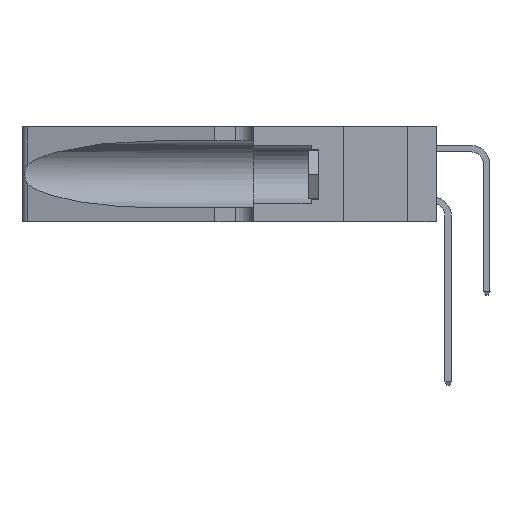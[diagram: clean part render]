
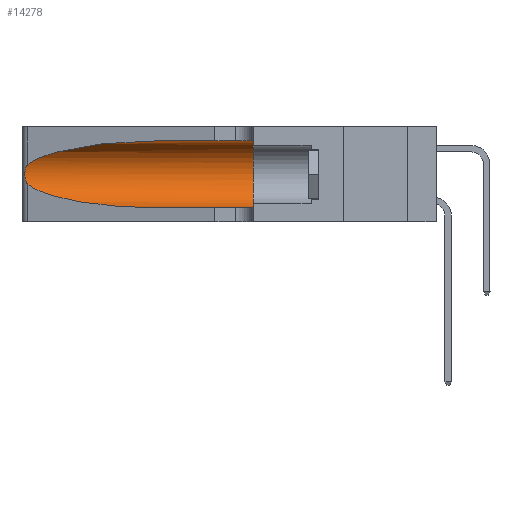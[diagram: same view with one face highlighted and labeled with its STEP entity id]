
A CAD part, left-side view. The second image highlights one B-rep face of the part: STEP entity #14278.
In plain terms, the highlighted cylindrical face has radius 3.308 mm (diameter 6.617 mm), a partial arc.
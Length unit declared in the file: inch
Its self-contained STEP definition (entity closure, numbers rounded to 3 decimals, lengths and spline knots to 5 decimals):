
#244 = CARTESIAN_POINT ( 'NONE',  ( 0.1305, 0.35, 0.31525 ) ) ;
#509 = CARTESIAN_POINT ( 'NONE',  ( 0.1305, 1.61858, 0.31525 ) ) ;
#1307 = CARTESIAN_POINT ( 'NONE',  ( 0.25787, 1.23484, 0.2124 ) ) ;
#2764 = CIRCLE ( 'NONE', #5358, 0.13025 ) ;
#2987 = CARTESIAN_POINT ( 'NONE',  ( 0.25487, 1.22718, 0.22369 ) ) ;
#3011 = DIRECTION ( 'NONE',  ( 0., 0., -1. ) ) ;
#3048 = DIRECTION ( 'NONE',  ( 0., -1., 0. ) ) ;
#3838 = CARTESIAN_POINT ( 'NONE',  ( 0.26018, 1.23835, 0.19895 ) ) ;
#4254 = VECTOR ( 'NONE', #31421, 39.37008 ) ;
#5358 = AXIS2_PLACEMENT_3D ( 'NONE', #22329, #7317, #24875 ) ;
#5828 = CARTESIAN_POINT ( 'NONE',  ( 0.1305, 0.72297, 0.05475 ) ) ;
#6239 = VERTEX_POINT ( 'NONE', #31519 ) ;
#6357 = CARTESIAN_POINT ( 'NONE',  ( 0.26075, 1.23896, 0.178 ) ) ;
#7317 = DIRECTION ( 'NONE',  ( 0., 1., 0. ) ) ;
#7642 = ORIENTED_EDGE ( 'NONE', *, *, #16237, .T. ) ;
#8105 = CARTESIAN_POINT ( 'NONE',  ( 0.25487, 1.22718, 0.14631 ) ) ;
#8329 = VERTEX_POINT ( 'NONE', #24674 ) ;
#8758 = ORIENTED_EDGE ( 'NONE', *, *, #21262, .T. ) ;
#8881 = CARTESIAN_POINT ( 'NONE',  ( 0.25856, 1.23593, 0.16098 ) ) ;
#9462 = EDGE_CURVE ( 'NONE', #8329, #6239, #12235, .T. ) ;
#9701 = VERTEX_POINT ( 'NONE', #27250 ) ;
#10558 = DIRECTION ( 'NONE',  ( 0., -1., 0. ) ) ;
#10921 = AXIS2_PLACEMENT_3D ( 'NONE', #30555, #10558, #3011 ) ;
#11334 = ORIENTED_EDGE ( 'NONE', *, *, #9462, .T. ) ;
#11382 = CARTESIAN_POINT ( 'NONE',  ( 0.25639, 1.23186, 0.15144 ) ) ;
#11475 = ORIENTED_EDGE ( 'NONE', *, *, #11864, .F. ) ;
#11864 = EDGE_CURVE ( 'NONE', #13810, #26033, #22912, .T. ) ;
#12235 = B_SPLINE_CURVE_WITH_KNOTS ( 'NONE', 3,
 ( #23805, #13775, #16309, #1307, #18819, #3838, #21334, #6357, #23907, #8881, #26421, #11382, #28908, #13889 ),
 .UNSPECIFIED., .F., .F.,
 ( 4, 2, 2, 2, 2, 2, 4 ),
 ( 0., 0.00027, 0.00053, 0.00107, 0.0016, 0.00187, 0.00214 ),
 .UNSPECIFIED. ) ;
#12995 = CARTESIAN_POINT ( 'NONE',  ( 0.1305, 0.72297, 0.05475 ) ) ;
#13253 = CARTESIAN_POINT ( 'NONE',  ( 0.2373, 1.15595, 0.08982 ) ) ;
#13583 = VERTEX_POINT ( 'NONE', #12995 ) ;
#13775 = CARTESIAN_POINT ( 'NONE',  ( 0.25555, 1.22994, 0.2215 ) ) ;
#13810 = VERTEX_POINT ( 'NONE', #31344 ) ;
#13889 = CARTESIAN_POINT ( 'NONE',  ( 0.25487, 1.22718, 0.14631 ) ) ;
#13932 = CARTESIAN_POINT ( 'NONE',  ( 0.1305, 1.61858, 0.05475 ) ) ;
#13985 = ORIENTED_EDGE ( 'NONE', *, *, #19666, .T. ) ;
#14208 = EDGE_LOOP ( 'NONE', ( #7642, #11334, #13985, #8758, #28251, #11475 ) ) ;
#14278 = ADVANCED_FACE ( 'NONE', ( #30963 ), #22782, .F. ) ;
#16237 = EDGE_CURVE ( 'NONE', #13810, #8329, #27312, .T. ) ;
#16309 = CARTESIAN_POINT ( 'NONE',  ( 0.25639, 1.23184, 0.21858 ) ) ;
#17976 = CARTESIAN_POINT ( 'NONE',  ( 0.2373, 1.15595, 0.28018 ) ) ;
#18819 = CARTESIAN_POINT ( 'NONE',  ( 0.25854, 1.2359, 0.20912 ) ) ;
#19123 = LINE ( 'NONE', #13932, #4254 ) ;
#19666 = EDGE_CURVE ( 'NONE', #6239, #13583, #21480, .T. ) ;
#19986 = EDGE_CURVE ( 'NONE', #26033, #9701, #2764, .T. ) ;
#20775 = CARTESIAN_POINT ( 'NONE',  ( 0.18966, 0.96281, 0.05475 ) ) ;
#21262 = EDGE_CURVE ( 'NONE', #13583, #9701, #19123, .T. ) ;
#21334 = CARTESIAN_POINT ( 'NONE',  ( 0.26075, 1.23896, 0.19203 ) ) ;
#21480 =( BOUNDED_CURVE ( )  B_SPLINE_CURVE ( 3, ( #8105, #13253, #20775, #5828 ),
 .UNSPECIFIED., .F., .F. ) 
 B_SPLINE_CURVE_WITH_KNOTS ( ( 4, 4 ),
 ( 3.44316, 4.71239 ),
 .UNSPECIFIED. ) 
 CURVE ( )  GEOMETRIC_REPRESENTATION_ITEM ( )  RATIONAL_B_SPLINE_CURVE ( ( 1., 0.87, 0.87, 1. ) ) 
 REPRESENTATION_ITEM ( '' )  );
#22329 = CARTESIAN_POINT ( 'NONE',  ( 0.1305, 0.35, 0.185 ) ) ;
#22782 = CYLINDRICAL_SURFACE ( 'NONE', #10921, 0.13025 ) ;
#22912 = LINE ( 'NONE', #509, #28781 ) ;
#23805 = CARTESIAN_POINT ( 'NONE',  ( 0.25487, 1.22718, 0.22369 ) ) ;
#23907 = CARTESIAN_POINT ( 'NONE',  ( 0.26017, 1.23833, 0.17102 ) ) ;
#24674 = CARTESIAN_POINT ( 'NONE',  ( 0.25487, 1.22718, 0.22369 ) ) ;
#24875 = DIRECTION ( 'NONE',  ( 0., 0., 1. ) ) ;
#25437 = CARTESIAN_POINT ( 'NONE',  ( 0.18966, 0.96281, 0.31525 ) ) ;
#26033 = VERTEX_POINT ( 'NONE', #244 ) ;
#26421 = CARTESIAN_POINT ( 'NONE',  ( 0.25789, 1.23486, 0.15765 ) ) ;
#27250 = CARTESIAN_POINT ( 'NONE',  ( 0.1305, 0.35, 0.05475 ) ) ;
#27312 =( BOUNDED_CURVE ( )  B_SPLINE_CURVE ( 3, ( #30425, #25437, #17976, #2987 ),
 .UNSPECIFIED., .F., .F. ) 
 B_SPLINE_CURVE_WITH_KNOTS ( ( 4, 4 ),
 ( 1.5708, 2.84003 ),
 .UNSPECIFIED. ) 
 CURVE ( )  GEOMETRIC_REPRESENTATION_ITEM ( )  RATIONAL_B_SPLINE_CURVE ( ( 1., 0.87, 0.87, 1. ) ) 
 REPRESENTATION_ITEM ( '' )  );
#28251 = ORIENTED_EDGE ( 'NONE', *, *, #19986, .F. ) ;
#28781 = VECTOR ( 'NONE', #3048, 39.37008 ) ;
#28908 = CARTESIAN_POINT ( 'NONE',  ( 0.25555, 1.22993, 0.14849 ) ) ;
#30425 = CARTESIAN_POINT ( 'NONE',  ( 0.1305, 0.72297, 0.31525 ) ) ;
#30555 = CARTESIAN_POINT ( 'NONE',  ( 0.1305, 1.61858, 0.185 ) ) ;
#30963 = FACE_OUTER_BOUND ( 'NONE', #14208, .T. ) ;
#31344 = CARTESIAN_POINT ( 'NONE',  ( 0.1305, 0.72297, 0.31525 ) ) ;
#31421 = DIRECTION ( 'NONE',  ( 0., -1., 0. ) ) ;
#31519 = CARTESIAN_POINT ( 'NONE',  ( 0.25487, 1.22718, 0.14631 ) ) ;
